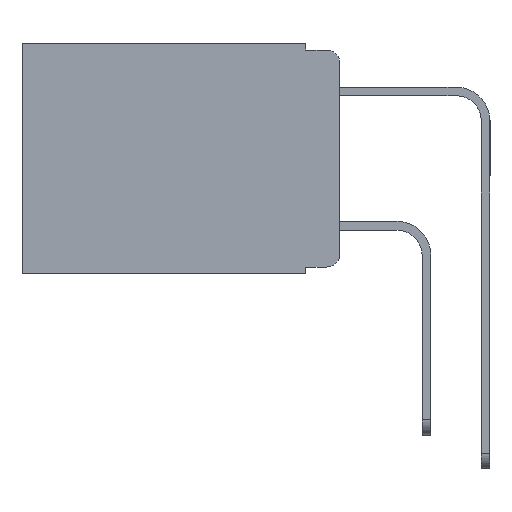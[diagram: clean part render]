
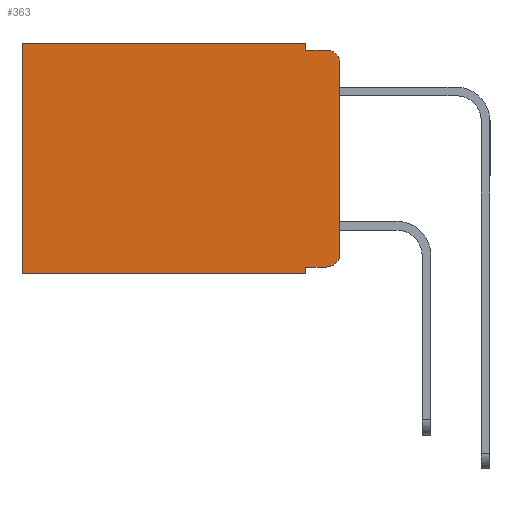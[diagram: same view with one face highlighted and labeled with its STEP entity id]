
A CAD part, left-side view. The second image highlights one B-rep face of the part: STEP entity #363.
In plain terms, the highlighted planar face has unit normal (-1, 0, 0).
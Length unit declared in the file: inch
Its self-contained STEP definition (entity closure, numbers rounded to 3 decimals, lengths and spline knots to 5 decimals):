
#363 = ADVANCED_FACE ( 'NONE', ( #6348 ), #8122, .F. ) ;
#419 = AXIS2_PLACEMENT_3D ( 'NONE', #3969, #8912, #517 ) ;
#466 = EDGE_LOOP ( 'NONE', ( #10187, #6994, #10118, #4969, #2009, #5570, #5970, #2281, #4764, #5642 ) ) ;
#517 = DIRECTION ( 'NONE',  ( 0., 0., -1. ) ) ;
#1010 = LINE ( 'NONE', #8724, #8305 ) ;
#1253 = CARTESIAN_POINT ( 'NONE',  ( 0.298, 0., 0. ) ) ;
#1580 = CARTESIAN_POINT ( 'NONE',  ( 0.298, 0.051, -0.01 ) ) ;
#1781 = CARTESIAN_POINT ( 'NONE',  ( 0.298, 0., 0. ) ) ;
#1978 = VERTEX_POINT ( 'NONE', #8058 ) ;
#2009 = ORIENTED_EDGE ( 'NONE', *, *, #4686, .T. ) ;
#2088 = VECTOR ( 'NONE', #12000, 39.37008 ) ;
#2148 = VERTEX_POINT ( 'NONE', #9683 ) ;
#2178 = DIRECTION ( 'NONE',  ( -1., 0., 0. ) ) ;
#2281 = ORIENTED_EDGE ( 'NONE', *, *, #4138, .F. ) ;
#2309 = VERTEX_POINT ( 'NONE', #8589 ) ;
#2379 = DIRECTION ( 'NONE',  ( 0., -1., 0. ) ) ;
#2391 = DIRECTION ( 'NONE',  ( 0., 0., -1. ) ) ;
#2426 = CIRCLE ( 'NONE', #8631, 0.02 ) ;
#2481 = DIRECTION ( 'NONE',  ( 0., 0., -1. ) ) ;
#2839 = DIRECTION ( 'NONE',  ( 0., 1., 0. ) ) ;
#3078 = CARTESIAN_POINT ( 'NONE',  ( 0.298, 0.473, 0. ) ) ;
#3603 = EDGE_CURVE ( 'NONE', #6982, #2309, #2426, .T. ) ;
#3969 = CARTESIAN_POINT ( 'NONE',  ( 0.298, 0.02, -0.03 ) ) ;
#4034 = LINE ( 'NONE', #1781, #4356 ) ;
#4138 = EDGE_CURVE ( 'NONE', #8037, #7522, #9009, .T. ) ;
#4356 = VECTOR ( 'NONE', #2839, 39.37008 ) ;
#4467 = CARTESIAN_POINT ( 'NONE',  ( 0.298, 0.051, 0. ) ) ;
#4499 = EDGE_CURVE ( 'NONE', #8037, #6982, #11674, .T. ) ;
#4612 = EDGE_CURVE ( 'NONE', #9075, #2148, #4953, .T. ) ;
#4686 = EDGE_CURVE ( 'NONE', #7086, #5732, #4034, .T. ) ;
#4690 = LINE ( 'NONE', #3078, #2088 ) ;
#4759 = DIRECTION ( 'NONE',  ( 0., 0., -1. ) ) ;
#4764 = ORIENTED_EDGE ( 'NONE', *, *, #4499, .T. ) ;
#4953 = CIRCLE ( 'NONE', #419, 0.02 ) ;
#4969 = ORIENTED_EDGE ( 'NONE', *, *, #10879, .F. ) ;
#5087 = CARTESIAN_POINT ( 'NONE',  ( 0.298, 0.051, 0. ) ) ;
#5271 = LINE ( 'NONE', #1253, #7387 ) ;
#5570 = ORIENTED_EDGE ( 'NONE', *, *, #11420, .T. ) ;
#5642 = ORIENTED_EDGE ( 'NONE', *, *, #3603, .T. ) ;
#5732 = VERTEX_POINT ( 'NONE', #8806 ) ;
#5970 = ORIENTED_EDGE ( 'NONE', *, *, #11619, .F. ) ;
#6044 = DIRECTION ( 'NONE',  ( 0., 1., 0. ) ) ;
#6348 = FACE_OUTER_BOUND ( 'NONE', #466, .T. ) ;
#6529 = VECTOR ( 'NONE', #7165, 39.37008 ) ;
#6943 = CARTESIAN_POINT ( 'NONE',  ( 0.298, 0., -0.03 ) ) ;
#6982 = VERTEX_POINT ( 'NONE', #10828 ) ;
#6994 = ORIENTED_EDGE ( 'NONE', *, *, #4612, .T. ) ;
#7048 = VECTOR ( 'NONE', #2379, 39.37008 ) ;
#7086 = VERTEX_POINT ( 'NONE', #4467 ) ;
#7123 = CARTESIAN_POINT ( 'NONE',  ( 0.298, 0.051, 0. ) ) ;
#7165 = DIRECTION ( 'NONE',  ( 0., -1., 0. ) ) ;
#7387 = VECTOR ( 'NONE', #2391, 39.37008 ) ;
#7522 = VERTEX_POINT ( 'NONE', #10400 ) ;
#8037 = VERTEX_POINT ( 'NONE', #10126 ) ;
#8058 = CARTESIAN_POINT ( 'NONE',  ( 0.298, 0.473, -0.343 ) ) ;
#8122 = PLANE ( 'NONE',  #10715 ) ;
#8264 = DIRECTION ( 'NONE',  ( 0., 0., -1. ) ) ;
#8305 = VECTOR ( 'NONE', #6044, 39.37008 ) ;
#8589 = CARTESIAN_POINT ( 'NONE',  ( 0.298, 0., -0.313 ) ) ;
#8631 = AXIS2_PLACEMENT_3D ( 'NONE', #12078, #2178, #8264 ) ;
#8724 = CARTESIAN_POINT ( 'NONE',  ( 0.298, 0., -0.343 ) ) ;
#8726 = VECTOR ( 'NONE', #4759, 39.37008 ) ;
#8806 = CARTESIAN_POINT ( 'NONE',  ( 0.298, 0.473, 0. ) ) ;
#8890 = LINE ( 'NONE', #10631, #6529 ) ;
#8912 = DIRECTION ( 'NONE',  ( -1., 0., 0. ) ) ;
#9009 = LINE ( 'NONE', #5087, #8726 ) ;
#9075 = VERTEX_POINT ( 'NONE', #6943 ) ;
#9178 = LINE ( 'NONE', #7123, #11191 ) ;
#9683 = CARTESIAN_POINT ( 'NONE',  ( 0.298, 0.02, -0.01 ) ) ;
#10118 = ORIENTED_EDGE ( 'NONE', *, *, #10945, .F. ) ;
#10126 = CARTESIAN_POINT ( 'NONE',  ( 0.298, 0.051, -0.333 ) ) ;
#10187 = ORIENTED_EDGE ( 'NONE', *, *, #10825, .F. ) ;
#10400 = CARTESIAN_POINT ( 'NONE',  ( 0.298, 0.051, -0.343 ) ) ;
#10423 = CARTESIAN_POINT ( 'NONE',  ( 0.298, 0., 0. ) ) ;
#10542 = DIRECTION ( 'NONE',  ( 1., 0., 0. ) ) ;
#10631 = CARTESIAN_POINT ( 'NONE',  ( 0.298, 0.051, -0.01 ) ) ;
#10679 = CARTESIAN_POINT ( 'NONE',  ( 0.298, 0.051, -0.333 ) ) ;
#10715 = AXIS2_PLACEMENT_3D ( 'NONE', #10423, #10542, #11386 ) ;
#10825 = EDGE_CURVE ( 'NONE', #9075, #2309, #5271, .T. ) ;
#10828 = CARTESIAN_POINT ( 'NONE',  ( 0.298, 0.02, -0.333 ) ) ;
#10879 = EDGE_CURVE ( 'NONE', #7086, #11984, #9178, .T. ) ;
#10945 = EDGE_CURVE ( 'NONE', #11984, #2148, #8890, .T. ) ;
#11191 = VECTOR ( 'NONE', #2481, 39.37008 ) ;
#11386 = DIRECTION ( 'NONE',  ( 0., 0., -1. ) ) ;
#11420 = EDGE_CURVE ( 'NONE', #5732, #1978, #4690, .T. ) ;
#11619 = EDGE_CURVE ( 'NONE', #7522, #1978, #1010, .T. ) ;
#11674 = LINE ( 'NONE', #10679, #7048 ) ;
#11984 = VERTEX_POINT ( 'NONE', #1580 ) ;
#12000 = DIRECTION ( 'NONE',  ( 0., 0., -1. ) ) ;
#12078 = CARTESIAN_POINT ( 'NONE',  ( 0.298, 0.02, -0.313 ) ) ;
